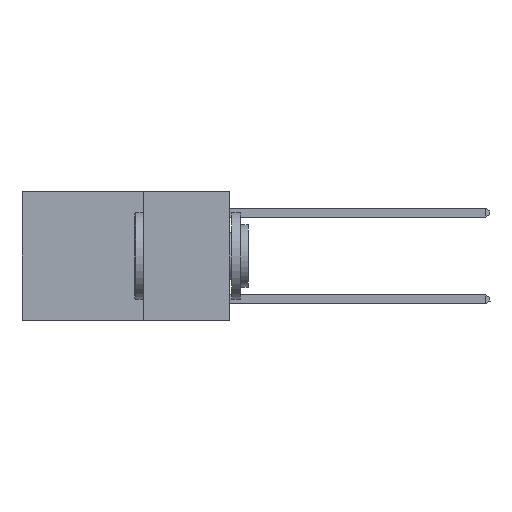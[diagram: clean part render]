
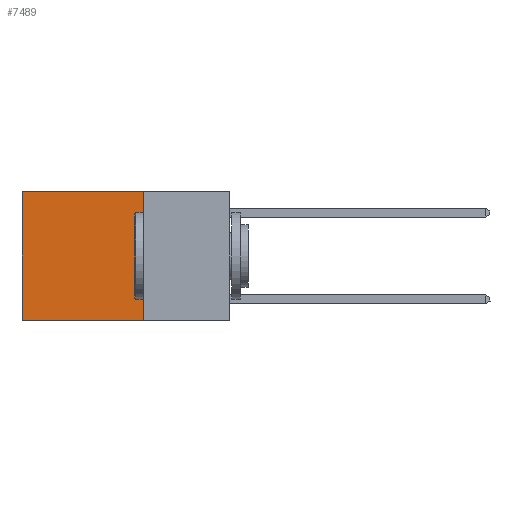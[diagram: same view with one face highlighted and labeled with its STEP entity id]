
A CAD part, left-side view. The second image highlights one B-rep face of the part: STEP entity #7489.
In plain terms, the highlighted planar face has unit normal (-1, 0, 0).
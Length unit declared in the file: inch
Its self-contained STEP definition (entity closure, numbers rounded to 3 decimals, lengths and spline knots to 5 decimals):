
#37 = CARTESIAN_POINT ( 'NONE',  ( 0.2625, 0.25, 0. ) ) ;
#377 = LINE ( 'NONE', #13678, #11754 ) ;
#776 = CARTESIAN_POINT ( 'NONE',  ( 0.2625, 0.25, -0.37 ) ) ;
#960 = DIRECTION ( 'NONE',  ( 0., 1., 0. ) ) ;
#1431 = DIRECTION ( 'NONE',  ( 0., 1., 0. ) ) ;
#1450 = EDGE_CURVE ( 'NONE', #16695, #8609, #12426, .T. ) ;
#2298 = CARTESIAN_POINT ( 'NONE',  ( 0.2625, 0.25, 0. ) ) ;
#2317 = VERTEX_POINT ( 'NONE', #37 ) ;
#2770 = EDGE_CURVE ( 'NONE', #2317, #7838, #16274, .T. ) ;
#3397 = CARTESIAN_POINT ( 'NONE',  ( 0.2625, 0.25, 0. ) ) ;
#3540 = ORIENTED_EDGE ( 'NONE', *, *, #7266, .F. ) ;
#3680 = ORIENTED_EDGE ( 'NONE', *, *, #2770, .T. ) ;
#4254 = VECTOR ( 'NONE', #960, 39.37008 ) ;
#4375 = AXIS2_PLACEMENT_3D ( 'NONE', #3397, #10203, #4836 ) ;
#4836 = DIRECTION ( 'NONE',  ( 0., 0., -1. ) ) ;
#4904 = ORIENTED_EDGE ( 'NONE', *, *, #14351, .T. ) ;
#5628 = LINE ( 'NONE', #12218, #17409 ) ;
#6157 = PLANE ( 'NONE',  #4375 ) ;
#7266 = EDGE_CURVE ( 'NONE', #2317, #16695, #5628, .T. ) ;
#7489 = ADVANCED_FACE ( 'NONE', ( #11834 ), #6157, .F. ) ;
#7838 = VERTEX_POINT ( 'NONE', #9896 ) ;
#8311 = CARTESIAN_POINT ( 'NONE',  ( 0.2625, 0.25, -0.37 ) ) ;
#8609 = VERTEX_POINT ( 'NONE', #17057 ) ;
#9545 = DIRECTION ( 'NONE',  ( 0., 0., -1. ) ) ;
#9896 = CARTESIAN_POINT ( 'NONE',  ( 0.2625, 0.6, 0. ) ) ;
#10203 = DIRECTION ( 'NONE',  ( 1., 0., 0. ) ) ;
#11754 = VECTOR ( 'NONE', #9545, 39.37008 ) ;
#11834 = FACE_OUTER_BOUND ( 'NONE', #12470, .T. ) ;
#12218 = CARTESIAN_POINT ( 'NONE',  ( 0.2625, 0.25, 0. ) ) ;
#12426 = LINE ( 'NONE', #8311, #16481 ) ;
#12470 = EDGE_LOOP ( 'NONE', ( #4904, #17436, #3540, #3680 ) ) ;
#13678 = CARTESIAN_POINT ( 'NONE',  ( 0.2625, 0.6, 0. ) ) ;
#14351 = EDGE_CURVE ( 'NONE', #7838, #8609, #377, .T. ) ;
#14997 = DIRECTION ( 'NONE',  ( 0., 0., -1. ) ) ;
#16274 = LINE ( 'NONE', #2298, #4254 ) ;
#16481 = VECTOR ( 'NONE', #1431, 39.37008 ) ;
#16695 = VERTEX_POINT ( 'NONE', #776 ) ;
#17057 = CARTESIAN_POINT ( 'NONE',  ( 0.2625, 0.6, -0.37 ) ) ;
#17409 = VECTOR ( 'NONE', #14997, 39.37008 ) ;
#17436 = ORIENTED_EDGE ( 'NONE', *, *, #1450, .F. ) ;
